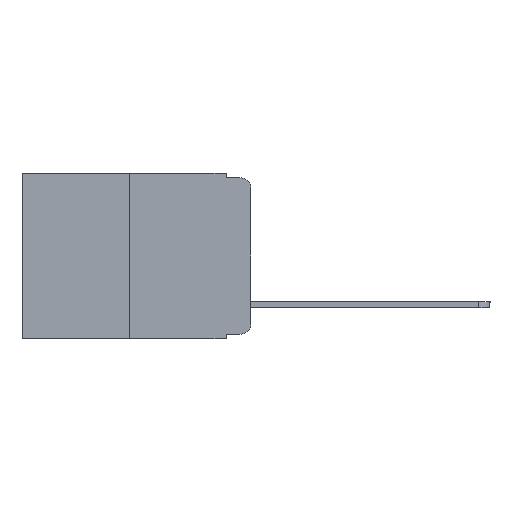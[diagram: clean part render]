
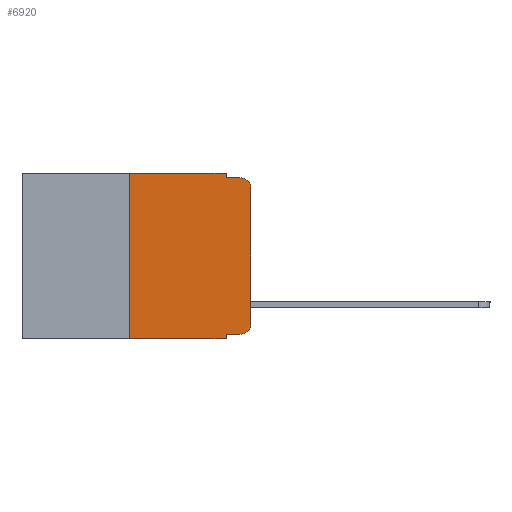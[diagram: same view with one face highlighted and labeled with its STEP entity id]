
A CAD part, left-side view. The second image highlights one B-rep face of the part: STEP entity #6920.
In plain terms, the highlighted planar face has unit normal (-1, 0, 0).
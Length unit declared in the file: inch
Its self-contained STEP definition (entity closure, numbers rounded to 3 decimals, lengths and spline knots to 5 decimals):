
#43 = FACE_OUTER_BOUND ( 'NONE', #3102, .T. ) ;
#71 = CARTESIAN_POINT ( 'NONE',  ( 0., 0.473, 0. ) ) ;
#99 = ORIENTED_EDGE ( 'NONE', *, *, #13115, .F. ) ;
#166 = VERTEX_POINT ( 'NONE', #4950 ) ;
#276 = CARTESIAN_POINT ( 'NONE',  ( 0., 0.051, -0.01 ) ) ;
#917 = LINE ( 'NONE', #7790, #2880 ) ;
#1035 = EDGE_CURVE ( 'NONE', #9549, #13158, #917, .T. ) ;
#1085 = CARTESIAN_POINT ( 'NONE',  ( 0., 0.473, -0.343 ) ) ;
#1279 = PLANE ( 'NONE',  #9424 ) ;
#1410 = CIRCLE ( 'NONE', #7514, 0.02 ) ;
#1440 = VERTEX_POINT ( 'NONE', #7916 ) ;
#1695 = DIRECTION ( 'NONE',  ( 0., 0., -1. ) ) ;
#1971 = VECTOR ( 'NONE', #11761, 39.37008 ) ;
#1992 = CARTESIAN_POINT ( 'NONE',  ( 0., 0.051, 0. ) ) ;
#2154 = CARTESIAN_POINT ( 'NONE',  ( 0., 0., -0.03 ) ) ;
#2644 = CARTESIAN_POINT ( 'NONE',  ( 0., 0.051, -0.333 ) ) ;
#2782 = VERTEX_POINT ( 'NONE', #14887 ) ;
#2880 = VECTOR ( 'NONE', #11372, 39.37008 ) ;
#3102 = EDGE_LOOP ( 'NONE', ( #6582, #3929, #5437, #12519, #99, #10510, #12394, #4030, #6899, #11123 ) ) ;
#3189 = VECTOR ( 'NONE', #7488, 39.37008 ) ;
#3496 = EDGE_CURVE ( 'NONE', #11489, #2782, #7432, .T. ) ;
#3584 = CARTESIAN_POINT ( 'NONE',  ( 0., 0.473, 0. ) ) ;
#3725 = EDGE_CURVE ( 'NONE', #166, #12538, #4466, .T. ) ;
#3803 = DIRECTION ( 'NONE',  ( 0., -1., 0. ) ) ;
#3853 = CARTESIAN_POINT ( 'NONE',  ( 0., 0.02, -0.03 ) ) ;
#3896 = EDGE_CURVE ( 'NONE', #11489, #12538, #10848, .T. ) ;
#3929 = ORIENTED_EDGE ( 'NONE', *, *, #9666, .T. ) ;
#4004 = CARTESIAN_POINT ( 'NONE',  ( 0., 0.02, -0.313 ) ) ;
#4030 = ORIENTED_EDGE ( 'NONE', *, *, #3896, .F. ) ;
#4466 = LINE ( 'NONE', #1085, #6116 ) ;
#4508 = DIRECTION ( 'NONE',  ( 0., 0., -1. ) ) ;
#4950 = CARTESIAN_POINT ( 'NONE',  ( 0., 0.25, -0.343 ) ) ;
#5010 = EDGE_CURVE ( 'NONE', #166, #9699, #7342, .T. ) ;
#5233 = DIRECTION ( 'NONE',  ( -1., 0., 0. ) ) ;
#5437 = ORIENTED_EDGE ( 'NONE', *, *, #5884, .F. ) ;
#5722 = DIRECTION ( 'NONE',  ( 1., 0., 0. ) ) ;
#5884 = EDGE_CURVE ( 'NONE', #7666, #1440, #12170, .T. ) ;
#6116 = VECTOR ( 'NONE', #13937, 39.37008 ) ;
#6137 = DIRECTION ( 'NONE',  ( -1., 0., 0. ) ) ;
#6582 = ORIENTED_EDGE ( 'NONE', *, *, #1035, .T. ) ;
#6899 = ORIENTED_EDGE ( 'NONE', *, *, #3496, .T. ) ;
#6920 = ADVANCED_FACE ( 'NONE', ( #43 ), #1279, .F. ) ;
#7111 = LINE ( 'NONE', #71, #9914 ) ;
#7118 = CARTESIAN_POINT ( 'NONE',  ( 0., 0.051, 0. ) ) ;
#7342 = LINE ( 'NONE', #13149, #3189 ) ;
#7432 = LINE ( 'NONE', #2644, #10975 ) ;
#7488 = DIRECTION ( 'NONE',  ( 0., 0., 1. ) ) ;
#7514 = AXIS2_PLACEMENT_3D ( 'NONE', #3853, #6137, #1695 ) ;
#7666 = VERTEX_POINT ( 'NONE', #8882 ) ;
#7790 = CARTESIAN_POINT ( 'NONE',  ( 0., 0., 0. ) ) ;
#7916 = CARTESIAN_POINT ( 'NONE',  ( 0., 0.02, -0.01 ) ) ;
#7999 = CARTESIAN_POINT ( 'NONE',  ( 0., 0.051, -0.343 ) ) ;
#8168 = VECTOR ( 'NONE', #4508, 39.37008 ) ;
#8308 = CARTESIAN_POINT ( 'NONE',  ( 0., 0.051, 0. ) ) ;
#8882 = CARTESIAN_POINT ( 'NONE',  ( 0., 0.051, -0.01 ) ) ;
#9424 = AXIS2_PLACEMENT_3D ( 'NONE', #3584, #5722, #13896 ) ;
#9462 = LINE ( 'NONE', #8308, #8168 ) ;
#9549 = VERTEX_POINT ( 'NONE', #11841 ) ;
#9666 = EDGE_CURVE ( 'NONE', #13158, #1440, #1410, .T. ) ;
#9699 = VERTEX_POINT ( 'NONE', #13621 ) ;
#9914 = VECTOR ( 'NONE', #14076, 39.37008 ) ;
#10510 = ORIENTED_EDGE ( 'NONE', *, *, #5010, .F. ) ;
#10848 = LINE ( 'NONE', #7118, #1971 ) ;
#10975 = VECTOR ( 'NONE', #12075, 39.37008 ) ;
#11123 = ORIENTED_EDGE ( 'NONE', *, *, #12823, .T. ) ;
#11372 = DIRECTION ( 'NONE',  ( 0., 0., 1. ) ) ;
#11489 = VERTEX_POINT ( 'NONE', #12581 ) ;
#11591 = EDGE_CURVE ( 'NONE', #14663, #7666, #9462, .T. ) ;
#11761 = DIRECTION ( 'NONE',  ( 0., 0., -1. ) ) ;
#11841 = CARTESIAN_POINT ( 'NONE',  ( 0., 0., -0.313 ) ) ;
#12075 = DIRECTION ( 'NONE',  ( 0., -1., 0. ) ) ;
#12170 = LINE ( 'NONE', #276, #15022 ) ;
#12342 = CIRCLE ( 'NONE', #13337, 0.02 ) ;
#12394 = ORIENTED_EDGE ( 'NONE', *, *, #3725, .T. ) ;
#12519 = ORIENTED_EDGE ( 'NONE', *, *, #11591, .F. ) ;
#12538 = VERTEX_POINT ( 'NONE', #7999 ) ;
#12581 = CARTESIAN_POINT ( 'NONE',  ( 0., 0.051, -0.333 ) ) ;
#12823 = EDGE_CURVE ( 'NONE', #2782, #9549, #12342, .T. ) ;
#13115 = EDGE_CURVE ( 'NONE', #9699, #14663, #7111, .T. ) ;
#13149 = CARTESIAN_POINT ( 'NONE',  ( 0., 0.25, 0. ) ) ;
#13158 = VERTEX_POINT ( 'NONE', #2154 ) ;
#13337 = AXIS2_PLACEMENT_3D ( 'NONE', #4004, #5233, #14534 ) ;
#13621 = CARTESIAN_POINT ( 'NONE',  ( 0., 0.25, 0. ) ) ;
#13896 = DIRECTION ( 'NONE',  ( 0., 0., -1. ) ) ;
#13937 = DIRECTION ( 'NONE',  ( 0., -1., 0. ) ) ;
#14076 = DIRECTION ( 'NONE',  ( 0., -1., 0. ) ) ;
#14534 = DIRECTION ( 'NONE',  ( 0., 0., -1. ) ) ;
#14663 = VERTEX_POINT ( 'NONE', #1992 ) ;
#14887 = CARTESIAN_POINT ( 'NONE',  ( 0., 0.02, -0.333 ) ) ;
#15022 = VECTOR ( 'NONE', #3803, 39.37008 ) ;
